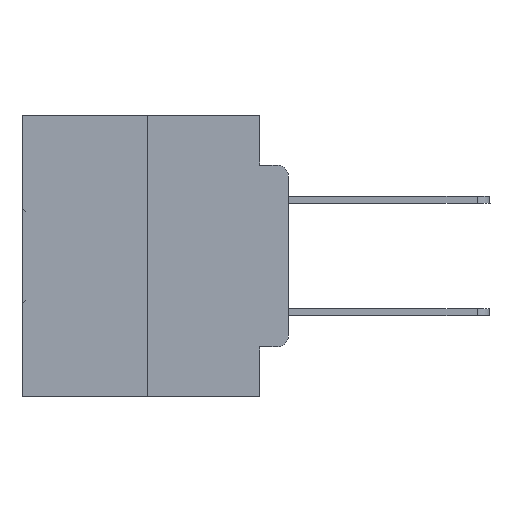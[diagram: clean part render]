
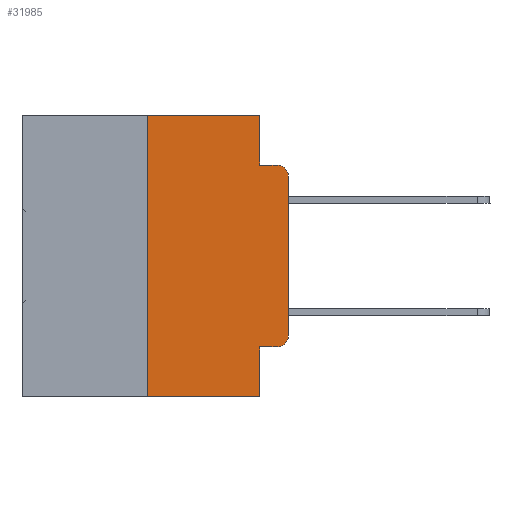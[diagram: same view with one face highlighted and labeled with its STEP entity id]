
A CAD part, left-side view. The second image highlights one B-rep face of the part: STEP entity #31985.
In plain terms, the highlighted planar face has unit normal (-1, 0, 0).
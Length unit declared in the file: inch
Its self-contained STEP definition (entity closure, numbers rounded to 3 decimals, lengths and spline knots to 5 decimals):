
#716 = VERTEX_POINT ( 'NONE', #28336 ) ;
#1909 = AXIS2_PLACEMENT_3D ( 'NONE', #8719, #26094, #11241 ) ;
#2099 = CARTESIAN_POINT ( 'NONE',  ( 0., 0.02, -0.0885 ) ) ;
#2414 = VERTEX_POINT ( 'NONE', #25260 ) ;
#3503 = ORIENTED_EDGE ( 'NONE', *, *, #29696, .T. ) ;
#3653 = DIRECTION ( 'NONE',  ( 0., 0., -1. ) ) ;
#3769 = CARTESIAN_POINT ( 'NONE',  ( 0., 0., 0. ) ) ;
#4056 = VECTOR ( 'NONE', #17837, 39.37008 ) ;
#4085 = EDGE_CURVE ( 'NONE', #15922, #2414, #10861, .T. ) ;
#4847 = LINE ( 'NONE', #30077, #4056 ) ;
#5574 = ORIENTED_EDGE ( 'NONE', *, *, #18161, .F. ) ;
#5621 = VECTOR ( 'NONE', #23870, 39.37008 ) ;
#5684 = DIRECTION ( 'NONE',  ( 0., 0., 1. ) ) ;
#5724 = VERTEX_POINT ( 'NONE', #18489 ) ;
#5836 = VECTOR ( 'NONE', #22737, 39.37008 ) ;
#6104 = VECTOR ( 'NONE', #14228, 39.37008 ) ;
#6455 = CARTESIAN_POINT ( 'NONE',  ( 0., 0.473, -0.5 ) ) ;
#6581 = ORIENTED_EDGE ( 'NONE', *, *, #26521, .F. ) ;
#7531 = VERTEX_POINT ( 'NONE', #31112 ) ;
#7585 = AXIS2_PLACEMENT_3D ( 'NONE', #29035, #14272, #31480 ) ;
#8305 = VECTOR ( 'NONE', #3653, 39.37008 ) ;
#8719 = CARTESIAN_POINT ( 'NONE',  ( 0., 0.02, -0.1085 ) ) ;
#9603 = EDGE_CURVE ( 'NONE', #31958, #5724, #14196, .T. ) ;
#10861 = LINE ( 'NONE', #3769, #28280 ) ;
#10961 = ORIENTED_EDGE ( 'NONE', *, *, #4085, .T. ) ;
#11241 = DIRECTION ( 'NONE',  ( 0., 0., -1. ) ) ;
#11646 = CIRCLE ( 'NONE', #1909, 0.02 ) ;
#11714 = CARTESIAN_POINT ( 'NONE',  ( 0., 0.25, 0. ) ) ;
#12146 = CARTESIAN_POINT ( 'NONE',  ( 0., 0.02, -0.4115 ) ) ;
#12334 = LINE ( 'NONE', #6455, #5621 ) ;
#12362 = VECTOR ( 'NONE', #15120, 39.37008 ) ;
#13721 = DIRECTION ( 'NONE',  ( 1., 0., 0. ) ) ;
#13776 = ORIENTED_EDGE ( 'NONE', *, *, #16934, .F. ) ;
#14196 = LINE ( 'NONE', #18695, #8305 ) ;
#14228 = DIRECTION ( 'NONE',  ( 0., 0., 1. ) ) ;
#14272 = DIRECTION ( 'NONE',  ( -1., 0., 0. ) ) ;
#14297 = VERTEX_POINT ( 'NONE', #2099 ) ;
#14386 = CARTESIAN_POINT ( 'NONE',  ( 0., 0.051, 0. ) ) ;
#15120 = DIRECTION ( 'NONE',  ( 0., -1., 0. ) ) ;
#15922 = VERTEX_POINT ( 'NONE', #22522 ) ;
#16307 = EDGE_CURVE ( 'NONE', #31101, #15922, #18271, .T. ) ;
#16934 = EDGE_CURVE ( 'NONE', #7531, #25366, #25955, .T. ) ;
#17170 = ORIENTED_EDGE ( 'NONE', *, *, #21501, .T. ) ;
#17323 = VECTOR ( 'NONE', #29846, 39.37008 ) ;
#17837 = DIRECTION ( 'NONE',  ( 0., -1., 0. ) ) ;
#18097 = LINE ( 'NONE', #14386, #17323 ) ;
#18161 = EDGE_CURVE ( 'NONE', #716, #21005, #18097, .T. ) ;
#18271 = CIRCLE ( 'NONE', #7585, 0.02 ) ;
#18489 = CARTESIAN_POINT ( 'NONE',  ( 0., 0.051, -0.0885 ) ) ;
#18547 = CARTESIAN_POINT ( 'NONE',  ( 0., 0.25, 0. ) ) ;
#18695 = CARTESIAN_POINT ( 'NONE',  ( 0., 0.051, 0. ) ) ;
#19650 = ORIENTED_EDGE ( 'NONE', *, *, #26898, .T. ) ;
#20522 = LINE ( 'NONE', #27412, #12362 ) ;
#21005 = VERTEX_POINT ( 'NONE', #26071 ) ;
#21501 = EDGE_CURVE ( 'NONE', #2414, #14297, #11646, .T. ) ;
#22383 = ORIENTED_EDGE ( 'NONE', *, *, #9603, .F. ) ;
#22522 = CARTESIAN_POINT ( 'NONE',  ( 0., 0., -0.3915 ) ) ;
#22737 = DIRECTION ( 'NONE',  ( 0., -1., 0. ) ) ;
#22753 = ORIENTED_EDGE ( 'NONE', *, *, #26432, .F. ) ;
#23379 = CARTESIAN_POINT ( 'NONE',  ( 0., 0.051, 0. ) ) ;
#23870 = DIRECTION ( 'NONE',  ( 0., -1., 0. ) ) ;
#24823 = ORIENTED_EDGE ( 'NONE', *, *, #16307, .T. ) ;
#25260 = CARTESIAN_POINT ( 'NONE',  ( 0., 0., -0.1085 ) ) ;
#25366 = VERTEX_POINT ( 'NONE', #18547 ) ;
#25955 = LINE ( 'NONE', #11714, #6104 ) ;
#26049 = PLANE ( 'NONE',  #26414 ) ;
#26071 = CARTESIAN_POINT ( 'NONE',  ( 0., 0.051, -0.5 ) ) ;
#26094 = DIRECTION ( 'NONE',  ( -1., 0., 0. ) ) ;
#26414 = AXIS2_PLACEMENT_3D ( 'NONE', #28502, #13721, #30936 ) ;
#26432 = EDGE_CURVE ( 'NONE', #5724, #14297, #20522, .T. ) ;
#26454 = LINE ( 'NONE', #30104, #5836 ) ;
#26521 = EDGE_CURVE ( 'NONE', #25366, #31958, #4847, .T. ) ;
#26898 = EDGE_CURVE ( 'NONE', #7531, #21005, #12334, .T. ) ;
#27412 = CARTESIAN_POINT ( 'NONE',  ( 0., 0.051, -0.0885 ) ) ;
#28280 = VECTOR ( 'NONE', #5684, 39.37008 ) ;
#28336 = CARTESIAN_POINT ( 'NONE',  ( 0., 0.051, -0.4115 ) ) ;
#28502 = CARTESIAN_POINT ( 'NONE',  ( 0., 0.473, 0. ) ) ;
#29035 = CARTESIAN_POINT ( 'NONE',  ( 0., 0.02, -0.3915 ) ) ;
#29696 = EDGE_CURVE ( 'NONE', #716, #31101, #26454, .T. ) ;
#29846 = DIRECTION ( 'NONE',  ( 0., 0., -1. ) ) ;
#30077 = CARTESIAN_POINT ( 'NONE',  ( 0., 0.473, 0. ) ) ;
#30104 = CARTESIAN_POINT ( 'NONE',  ( 0., 0.051, -0.4115 ) ) ;
#30936 = DIRECTION ( 'NONE',  ( 0., 0., -1. ) ) ;
#31101 = VERTEX_POINT ( 'NONE', #12146 ) ;
#31112 = CARTESIAN_POINT ( 'NONE',  ( 0., 0.25, -0.5 ) ) ;
#31114 = FACE_OUTER_BOUND ( 'NONE', #31467, .T. ) ;
#31467 = EDGE_LOOP ( 'NONE', ( #10961, #17170, #22753, #22383, #6581, #13776, #19650, #5574, #3503, #24823 ) ) ;
#31480 = DIRECTION ( 'NONE',  ( 0., 0., -1. ) ) ;
#31958 = VERTEX_POINT ( 'NONE', #23379 ) ;
#31985 = ADVANCED_FACE ( 'NONE', ( #31114 ), #26049, .F. ) ;
